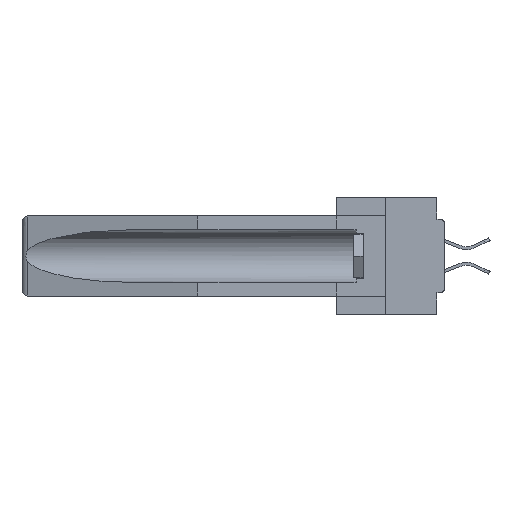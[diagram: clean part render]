
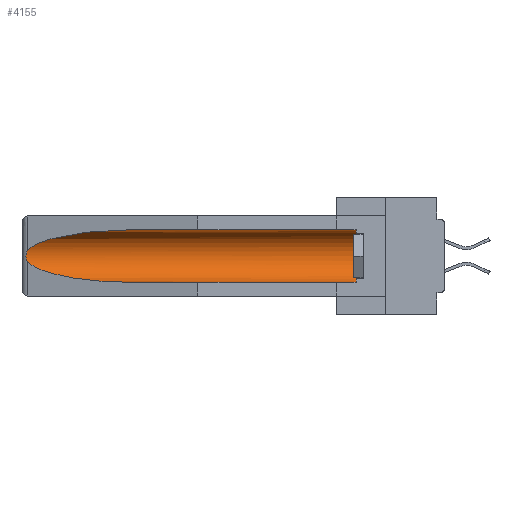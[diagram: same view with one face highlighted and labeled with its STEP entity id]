
A CAD part, left-side view. The second image highlights one B-rep face of the part: STEP entity #4155.
In plain terms, the highlighted cylindrical face has radius 2.857 mm (diameter 5.715 mm), a partial arc.
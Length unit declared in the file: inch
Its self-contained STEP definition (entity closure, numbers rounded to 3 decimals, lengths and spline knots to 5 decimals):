
#286 = CARTESIAN_POINT ( 'NONE',  ( 0.2675, 1.53308, -0.16763 ) ) ;
#437 = DIRECTION ( 'NONE',  ( 0., 1., 0. ) ) ;
#1548 = DIRECTION ( 'NONE',  ( 0., 1., 0. ) ) ;
#2707 = VERTEX_POINT ( 'NONE', #4108 ) ;
#3382 = VERTEX_POINT ( 'NONE', #34515 ) ;
#3616 = VECTOR ( 'NONE', #1548, 39.37008 ) ;
#3747 = CARTESIAN_POINT ( 'NONE',  ( 0.2673, 1.5327, -0.16383 ) ) ;
#4022 = CARTESIAN_POINT ( 'NONE',  ( 0.26654, 1.53092, -0.15636 ) ) ;
#4108 = CARTESIAN_POINT ( 'NONE',  ( 0.155, 1.07973, -0.284 ) ) ;
#4155 = ADVANCED_FACE ( 'NONE', ( #11885 ), #39476, .F. ) ;
#5342 = ORIENTED_EDGE ( 'NONE', *, *, #5566, .F. ) ;
#5421 = CARTESIAN_POINT ( 'NONE',  ( 0.155, 1.07973, -0.059 ) ) ;
#5566 = EDGE_CURVE ( 'NONE', #24343, #2707, #7574, .T. ) ;
#5998 = EDGE_CURVE ( 'NONE', #13270, #11581, #16474, .T. ) ;
#6339 = ORIENTED_EDGE ( 'NONE', *, *, #25969, .T. ) ;
#6711 = CARTESIAN_POINT ( 'NONE',  ( 0.155, 1.07973, -0.059 ) ) ;
#7172 = CARTESIAN_POINT ( 'NONE',  ( 0.26655, 1.53094, -0.18657 ) ) ;
#7423 = EDGE_CURVE ( 'NONE', #3382, #34324, #20509, .T. ) ;
#7574 = LINE ( 'NONE', #40029, #3616 ) ;
#7757 = CARTESIAN_POINT ( 'NONE',  ( 0.155, 1.07973, -0.284 ) ) ;
#8631 = CARTESIAN_POINT ( 'NONE',  ( 0.25451, 1.48313, -0.09465 ) ) ;
#9541 = CIRCLE ( 'NONE', #23425, 0.1125 ) ;
#11581 = VERTEX_POINT ( 'NONE', #32586 ) ;
#11885 = FACE_OUTER_BOUND ( 'NONE', #16846, .T. ) ;
#12142 = CARTESIAN_POINT ( 'NONE',  ( 0.21114, 1.30732, -0.059 ) ) ;
#12513 = VECTOR ( 'NONE', #437, 39.37008 ) ;
#13270 = VERTEX_POINT ( 'NONE', #40537 ) ;
#13520 = CARTESIAN_POINT ( 'NONE',  ( 0.2675, 1.53308, -0.17534 ) ) ;
#13970 = CARTESIAN_POINT ( 'NONE',  ( 0.21114, 1.30732, -0.284 ) ) ;
#16221 = DIRECTION ( 'NONE',  ( 0., -1., 0. ) ) ;
#16360 = CARTESIAN_POINT ( 'NONE',  ( 0.155, 0.126, -0.1715 ) ) ;
#16474 = B_SPLINE_CURVE_WITH_KNOTS ( 'NONE', 3,
 ( #23222, #22665, #4022, #3747, #286, #13520, #36101, #7172, #26446, #29698 ),
 .UNSPECIFIED., .F., .F.,
 ( 4, 2, 2, 2, 4 ),
 ( 0., 0.00029, 0.00058, 0.00087, 0.00117 ),
 .UNSPECIFIED. ) ;
#16783 = DIRECTION ( 'NONE',  ( 0., 0., 1. ) ) ;
#16846 = EDGE_LOOP ( 'NONE', ( #34133, #27277, #6339, #5342, #29070, #38711 ) ) ;
#16919 = CARTESIAN_POINT ( 'NONE',  ( 0.155, -0.30754, -0.1715 ) ) ;
#17003 =( BOUNDED_CURVE ( )  B_SPLINE_CURVE ( 3, ( #5421, #12142, #8631, #37392 ),
 .UNSPECIFIED., .F., .T. ) 
 B_SPLINE_CURVE_WITH_KNOTS ( ( 4, 4 ),
 ( 4.71239, 6.08839 ),
 .UNSPECIFIED. ) 
 CURVE ( )  GEOMETRIC_REPRESENTATION_ITEM ( )  RATIONAL_B_SPLINE_CURVE ( ( 1., 0.848, 0.848, 1. ) ) 
 REPRESENTATION_ITEM ( '' )  );
#17481 = CARTESIAN_POINT ( 'NONE',  ( 0.25451, 1.48313, -0.24835 ) ) ;
#19563 = CARTESIAN_POINT ( 'NONE',  ( 0.155, 0.126, -0.284 ) ) ;
#19972 = DIRECTION ( 'NONE',  ( 0., 0., 1. ) ) ;
#20509 = LINE ( 'NONE', #32231, #12513 ) ;
#20538 = CARTESIAN_POINT ( 'NONE',  ( 0.26537, 1.52718, -0.19328 ) ) ;
#22665 = CARTESIAN_POINT ( 'NONE',  ( 0.26597, 1.52961, -0.15275 ) ) ;
#23222 = CARTESIAN_POINT ( 'NONE',  ( 0.26537, 1.52718, -0.14972 ) ) ;
#23425 = AXIS2_PLACEMENT_3D ( 'NONE', #16360, #16221, #19972 ) ;
#24343 = VERTEX_POINT ( 'NONE', #19563 ) ;
#25969 = EDGE_CURVE ( 'NONE', #11581, #2707, #30642, .T. ) ;
#26446 = CARTESIAN_POINT ( 'NONE',  ( 0.26597, 1.5296, -0.19026 ) ) ;
#27277 = ORIENTED_EDGE ( 'NONE', *, *, #5998, .T. ) ;
#29070 = ORIENTED_EDGE ( 'NONE', *, *, #37241, .T. ) ;
#29452 = DIRECTION ( 'NONE',  ( 0., 1., 0. ) ) ;
#29698 = CARTESIAN_POINT ( 'NONE',  ( 0.26537, 1.52718, -0.19328 ) ) ;
#30642 =( BOUNDED_CURVE ( )  B_SPLINE_CURVE ( 3, ( #20538, #17481, #13970, #7757 ),
 .UNSPECIFIED., .F., .F. ) 
 B_SPLINE_CURVE_WITH_KNOTS ( ( 4, 4 ),
 ( 0.1948, 1.5708 ),
 .UNSPECIFIED. ) 
 CURVE ( )  GEOMETRIC_REPRESENTATION_ITEM ( )  RATIONAL_B_SPLINE_CURVE ( ( 1., 0.848, 0.848, 1. ) ) 
 REPRESENTATION_ITEM ( '' )  );
#32231 = CARTESIAN_POINT ( 'NONE',  ( 0.155, -0.30754, -0.059 ) ) ;
#32586 = CARTESIAN_POINT ( 'NONE',  ( 0.26537, 1.52718, -0.19328 ) ) ;
#34133 = ORIENTED_EDGE ( 'NONE', *, *, #36923, .T. ) ;
#34324 = VERTEX_POINT ( 'NONE', #6711 ) ;
#34515 = CARTESIAN_POINT ( 'NONE',  ( 0.155, 0.126, -0.059 ) ) ;
#36101 = CARTESIAN_POINT ( 'NONE',  ( 0.2673, 1.53269, -0.17917 ) ) ;
#36923 = EDGE_CURVE ( 'NONE', #34324, #13270, #17003, .T. ) ;
#37241 = EDGE_CURVE ( 'NONE', #24343, #3382, #9541, .T. ) ;
#37392 = CARTESIAN_POINT ( 'NONE',  ( 0.26537, 1.52718, -0.14972 ) ) ;
#38711 = ORIENTED_EDGE ( 'NONE', *, *, #7423, .T. ) ;
#38997 = AXIS2_PLACEMENT_3D ( 'NONE', #16919, #29452, #16783 ) ;
#39476 = CYLINDRICAL_SURFACE ( 'NONE', #38997, 0.1125 ) ;
#40029 = CARTESIAN_POINT ( 'NONE',  ( 0.155, -0.30754, -0.284 ) ) ;
#40537 = CARTESIAN_POINT ( 'NONE',  ( 0.26537, 1.52718, -0.14972 ) ) ;
